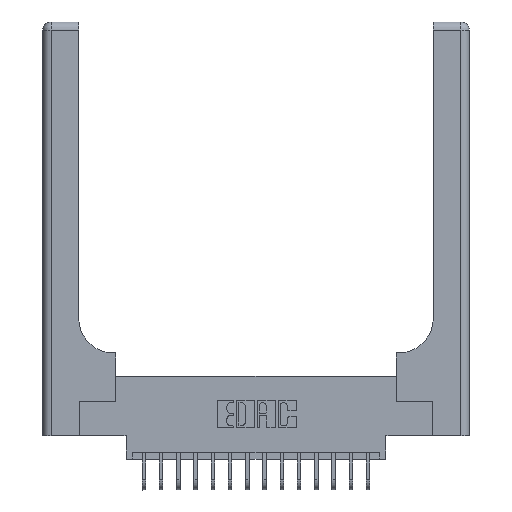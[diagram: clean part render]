
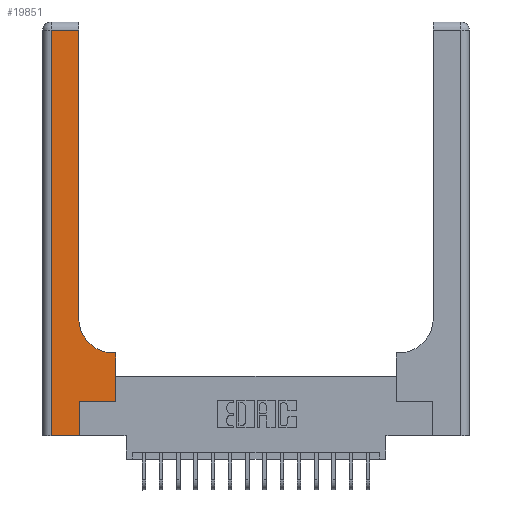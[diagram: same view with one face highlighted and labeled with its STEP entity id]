
A CAD part, top view. The second image highlights one B-rep face of the part: STEP entity #19851.
In plain terms, the highlighted planar face has unit normal (0, 0, 1).
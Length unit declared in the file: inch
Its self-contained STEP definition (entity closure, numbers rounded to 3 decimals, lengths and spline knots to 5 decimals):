
#121 = CARTESIAN_POINT ( 'NONE',  ( 0.26, 0.85, 0.37 ) ) ;
#629 = ORIENTED_EDGE ( 'NONE', *, *, #19581, .T. ) ;
#962 = DIRECTION ( 'NONE',  ( 0., 1., 0. ) ) ;
#1040 = VERTEX_POINT ( 'NONE', #18823 ) ;
#1046 = VERTEX_POINT ( 'NONE', #11423 ) ;
#1057 = EDGE_CURVE ( 'NONE', #11528, #5152, #16317, .T. ) ;
#1485 = DIRECTION ( 'NONE',  ( 0., 1., 0. ) ) ;
#1528 = EDGE_CURVE ( 'NONE', #11303, #11528, #19661, .T. ) ;
#2090 = CARTESIAN_POINT ( 'NONE',  ( 0., 3., 0.37 ) ) ;
#2591 = AXIS2_PLACEMENT_3D ( 'NONE', #14435, #15984, #19003 ) ;
#2659 = EDGE_CURVE ( 'NONE', #19055, #1046, #13107, .T. ) ;
#3245 = CARTESIAN_POINT ( 'NONE',  ( 0.51, 0.6, 0.37 ) ) ;
#3836 = ORIENTED_EDGE ( 'NONE', *, *, #1057, .T. ) ;
#3860 = VERTEX_POINT ( 'NONE', #121 ) ;
#3969 = CARTESIAN_POINT ( 'NONE',  ( 0.06, 2.94, 0.37 ) ) ;
#4034 = CARTESIAN_POINT ( 'NONE',  ( 0.06, 0., 0.37 ) ) ;
#4676 = VECTOR ( 'NONE', #12047, 39.37008 ) ;
#4725 = VECTOR ( 'NONE', #19525, 39.37008 ) ;
#4884 = VECTOR ( 'NONE', #13561, 39.37008 ) ;
#5152 = VERTEX_POINT ( 'NONE', #4034 ) ;
#5276 = AXIS2_PLACEMENT_3D ( 'NONE', #2090, #8273, #19029 ) ;
#5289 = ORIENTED_EDGE ( 'NONE', *, *, #11485, .T. ) ;
#5808 = EDGE_CURVE ( 'NONE', #3860, #11303, #18370, .T. ) ;
#6067 = EDGE_CURVE ( 'NONE', #5152, #7965, #11650, .T. ) ;
#6694 = PLANE ( 'NONE',  #5276 ) ;
#6889 = VECTOR ( 'NONE', #1485, 39.37008 ) ;
#7451 = LINE ( 'NONE', #16063, #8217 ) ;
#7965 = VERTEX_POINT ( 'NONE', #10962 ) ;
#8217 = VECTOR ( 'NONE', #14644, 39.37008 ) ;
#8273 = DIRECTION ( 'NONE',  ( 0., 0., -1. ) ) ;
#8699 = EDGE_CURVE ( 'NONE', #1046, #13902, #7451, .T. ) ;
#8794 = VECTOR ( 'NONE', #18612, 39.37008 ) ;
#9070 = ORIENTED_EDGE ( 'NONE', *, *, #1528, .T. ) ;
#9820 = DIRECTION ( 'NONE',  ( 0., -1., 0. ) ) ;
#10218 = CARTESIAN_POINT ( 'NONE',  ( 0., 0., 0.37 ) ) ;
#10843 = CIRCLE ( 'NONE', #2591, 0.25 ) ;
#10962 = CARTESIAN_POINT ( 'NONE',  ( 0.265, 0., 0.37 ) ) ;
#11303 = VERTEX_POINT ( 'NONE', #12267 ) ;
#11423 = CARTESIAN_POINT ( 'NONE',  ( 0.528, 0.6, 0.37 ) ) ;
#11485 = EDGE_CURVE ( 'NONE', #1040, #19055, #18177, .T. ) ;
#11528 = VERTEX_POINT ( 'NONE', #3969 ) ;
#11650 = LINE ( 'NONE', #10218, #4884 ) ;
#12047 = DIRECTION ( 'NONE',  ( 0., 1., 0. ) ) ;
#12267 = CARTESIAN_POINT ( 'NONE',  ( 0.26, 2.94, 0.37 ) ) ;
#12419 = ORIENTED_EDGE ( 'NONE', *, *, #5808, .T. ) ;
#12676 = ORIENTED_EDGE ( 'NONE', *, *, #14716, .T. ) ;
#12802 = FACE_OUTER_BOUND ( 'NONE', #13283, .T. ) ;
#12909 = ORIENTED_EDGE ( 'NONE', *, *, #8699, .T. ) ;
#13107 = LINE ( 'NONE', #18397, #4676 ) ;
#13283 = EDGE_LOOP ( 'NONE', ( #12419, #9070, #3836, #14817, #629, #5289, #14670, #12909, #12676 ) ) ;
#13561 = DIRECTION ( 'NONE',  ( 1., 0., 0. ) ) ;
#13902 = VERTEX_POINT ( 'NONE', #3245 ) ;
#14167 = VECTOR ( 'NONE', #9820, 39.37008 ) ;
#14435 = CARTESIAN_POINT ( 'NONE',  ( 0.51, 0.85, 0.37 ) ) ;
#14447 = CARTESIAN_POINT ( 'NONE',  ( 0.265, 0.25, 0.37 ) ) ;
#14644 = DIRECTION ( 'NONE',  ( -1., 0., 0. ) ) ;
#14670 = ORIENTED_EDGE ( 'NONE', *, *, #2659, .T. ) ;
#14716 = EDGE_CURVE ( 'NONE', #13902, #3860, #10843, .T. ) ;
#14817 = ORIENTED_EDGE ( 'NONE', *, *, #6067, .T. ) ;
#15330 = CARTESIAN_POINT ( 'NONE',  ( 0.265, 0., 0.37 ) ) ;
#15902 = CARTESIAN_POINT ( 'NONE',  ( 0.528, 0.25, 0.37 ) ) ;
#15984 = DIRECTION ( 'NONE',  ( 0., 0., -1. ) ) ;
#16063 = CARTESIAN_POINT ( 'NONE',  ( 0.26, 0.6, 0.37 ) ) ;
#16317 = LINE ( 'NONE', #18885, #14167 ) ;
#16559 = LINE ( 'NONE', #15330, #6889 ) ;
#17982 = CARTESIAN_POINT ( 'NONE',  ( 0., 2.94, 0.37 ) ) ;
#18177 = LINE ( 'NONE', #14447, #8794 ) ;
#18370 = LINE ( 'NONE', #19456, #18872 ) ;
#18397 = CARTESIAN_POINT ( 'NONE',  ( 0.528, 0.25, 0.37 ) ) ;
#18612 = DIRECTION ( 'NONE',  ( 1., 0., 0. ) ) ;
#18823 = CARTESIAN_POINT ( 'NONE',  ( 0.265, 0.25, 0.37 ) ) ;
#18872 = VECTOR ( 'NONE', #962, 39.37008 ) ;
#18885 = CARTESIAN_POINT ( 'NONE',  ( 0.06, 3., 0.37 ) ) ;
#19003 = DIRECTION ( 'NONE',  ( 1., 0., 0. ) ) ;
#19029 = DIRECTION ( 'NONE',  ( -1., 0., 0. ) ) ;
#19055 = VERTEX_POINT ( 'NONE', #15902 ) ;
#19456 = CARTESIAN_POINT ( 'NONE',  ( 0.26, 3., 0.37 ) ) ;
#19525 = DIRECTION ( 'NONE',  ( -1., 0., 0. ) ) ;
#19581 = EDGE_CURVE ( 'NONE', #7965, #1040, #16559, .T. ) ;
#19661 = LINE ( 'NONE', #17982, #4725 ) ;
#19851 = ADVANCED_FACE ( 'NONE', ( #12802 ), #6694, .F. ) ;
